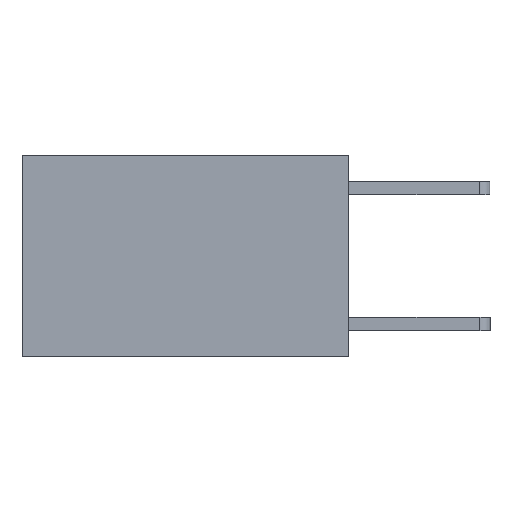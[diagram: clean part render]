
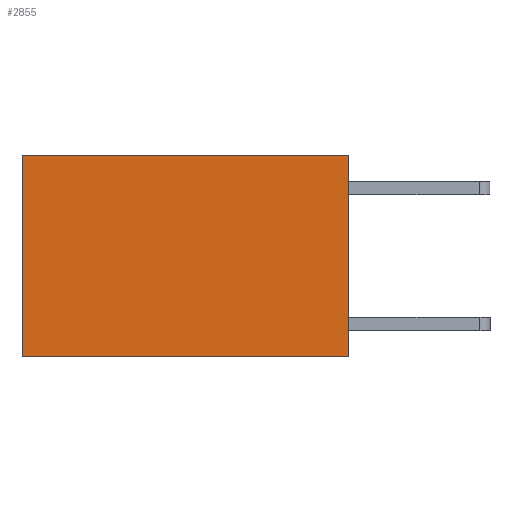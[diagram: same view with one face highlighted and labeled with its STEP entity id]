
A CAD part, left-side view. The second image highlights one B-rep face of the part: STEP entity #2855.
In plain terms, the highlighted planar face has unit normal (-1, 0, 0).
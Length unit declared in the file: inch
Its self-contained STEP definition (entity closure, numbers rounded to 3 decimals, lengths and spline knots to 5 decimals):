
#50 = DIRECTION ( 'NONE',  ( 0., 0., -1. ) ) ;
#216 = LINE ( 'NONE', #865, #3399 ) ;
#238 = CARTESIAN_POINT ( 'NONE',  ( 0.2625, 0., -0.37 ) ) ;
#242 = DIRECTION ( 'NONE',  ( 1., 0., 0. ) ) ;
#498 = DIRECTION ( 'NONE',  ( 0., 0., -1. ) ) ;
#815 = CARTESIAN_POINT ( 'NONE',  ( 0.2625, 0.6, -0.37 ) ) ;
#865 = CARTESIAN_POINT ( 'NONE',  ( 0.2625, 0., 0. ) ) ;
#895 = DIRECTION ( 'NONE',  ( 0., 1., 0. ) ) ;
#1055 = ORIENTED_EDGE ( 'NONE', *, *, #1813, .T. ) ;
#1588 = LINE ( 'NONE', #238, #6694 ) ;
#1813 = EDGE_CURVE ( 'NONE', #6194, #4813, #5687, .T. ) ;
#2264 = VECTOR ( 'NONE', #498, 39.37008 ) ;
#2525 = ORIENTED_EDGE ( 'NONE', *, *, #7528, .F. ) ;
#2762 = VECTOR ( 'NONE', #50, 39.37008 ) ;
#2855 = ADVANCED_FACE ( 'NONE', ( #4224 ), #5965, .F. ) ;
#3253 = CARTESIAN_POINT ( 'NONE',  ( 0.2625, 0., -0.37 ) ) ;
#3399 = VECTOR ( 'NONE', #895, 39.37008 ) ;
#3418 = EDGE_CURVE ( 'NONE', #3766, #6194, #216, .T. ) ;
#3430 = DIRECTION ( 'NONE',  ( 0., 1., 0. ) ) ;
#3510 = ORIENTED_EDGE ( 'NONE', *, *, #4884, .F. ) ;
#3624 = AXIS2_PLACEMENT_3D ( 'NONE', #4060, #242, #4716 ) ;
#3766 = VERTEX_POINT ( 'NONE', #6978 ) ;
#3852 = VERTEX_POINT ( 'NONE', #3253 ) ;
#4060 = CARTESIAN_POINT ( 'NONE',  ( 0.2625, 0., 0. ) ) ;
#4224 = FACE_OUTER_BOUND ( 'NONE', #4770, .T. ) ;
#4485 = LINE ( 'NONE', #4525, #2762 ) ;
#4525 = CARTESIAN_POINT ( 'NONE',  ( 0.2625, 0., 0. ) ) ;
#4716 = DIRECTION ( 'NONE',  ( 0., 0., -1. ) ) ;
#4770 = EDGE_LOOP ( 'NONE', ( #1055, #3510, #2525, #6056 ) ) ;
#4813 = VERTEX_POINT ( 'NONE', #815 ) ;
#4884 = EDGE_CURVE ( 'NONE', #3852, #4813, #1588, .T. ) ;
#4976 = CARTESIAN_POINT ( 'NONE',  ( 0.2625, 0.6, 0. ) ) ;
#5383 = CARTESIAN_POINT ( 'NONE',  ( 0.2625, 0.6, 0. ) ) ;
#5687 = LINE ( 'NONE', #4976, #2264 ) ;
#5965 = PLANE ( 'NONE',  #3624 ) ;
#6056 = ORIENTED_EDGE ( 'NONE', *, *, #3418, .T. ) ;
#6194 = VERTEX_POINT ( 'NONE', #5383 ) ;
#6694 = VECTOR ( 'NONE', #3430, 39.37008 ) ;
#6978 = CARTESIAN_POINT ( 'NONE',  ( 0.2625, 0., 0. ) ) ;
#7528 = EDGE_CURVE ( 'NONE', #3766, #3852, #4485, .T. ) ;
